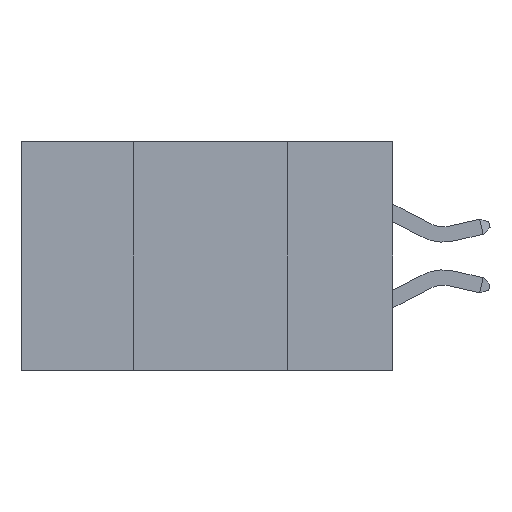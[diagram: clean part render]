
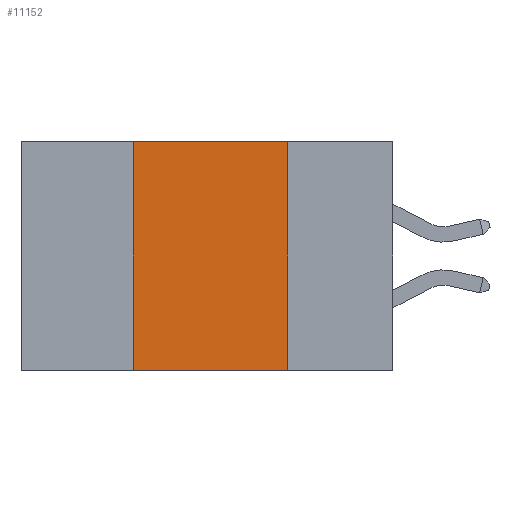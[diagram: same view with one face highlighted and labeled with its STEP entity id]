
A CAD part, left-side view. The second image highlights one B-rep face of the part: STEP entity #11152.
In plain terms, the highlighted planar face has unit normal (-1, 0, 0).
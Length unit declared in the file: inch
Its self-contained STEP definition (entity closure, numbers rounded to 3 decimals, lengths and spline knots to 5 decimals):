
#495 = DIRECTION ( 'NONE',  ( 0., 0., -1. ) ) ;
#962 = DIRECTION ( 'NONE',  ( 0., -1., 0. ) ) ;
#2037 = VECTOR ( 'NONE', #962, 39.37008 ) ;
#3722 = CARTESIAN_POINT ( 'NONE',  ( 0., 0.17, -0.37 ) ) ;
#4074 = ORIENTED_EDGE ( 'NONE', *, *, #23182, .F. ) ;
#4341 = VERTEX_POINT ( 'NONE', #3722 ) ;
#6495 = CARTESIAN_POINT ( 'NONE',  ( 0., 0.42, 0. ) ) ;
#6790 = LINE ( 'NONE', #6495, #18582 ) ;
#7471 = CARTESIAN_POINT ( 'NONE',  ( 0., 0.6, 0. ) ) ;
#7876 = VERTEX_POINT ( 'NONE', #23951 ) ;
#8425 = DIRECTION ( 'NONE',  ( 0., 0., -1. ) ) ;
#10256 = VERTEX_POINT ( 'NONE', #17752 ) ;
#10560 = LINE ( 'NONE', #11004, #13481 ) ;
#10595 = CARTESIAN_POINT ( 'NONE',  ( 0., 0.6, 0. ) ) ;
#11004 = CARTESIAN_POINT ( 'NONE',  ( 0., 0.6, -0.37 ) ) ;
#11152 = ADVANCED_FACE ( 'NONE', ( #28381 ), #21589, .F. ) ;
#11482 = CARTESIAN_POINT ( 'NONE',  ( 0., 0.17, 0. ) ) ;
#11497 = EDGE_CURVE ( 'NONE', #22914, #4341, #10560, .T. ) ;
#12917 = DIRECTION ( 'NONE',  ( 1., 0., 0. ) ) ;
#13481 = VECTOR ( 'NONE', #24138, 39.37008 ) ;
#13621 = EDGE_CURVE ( 'NONE', #7876, #10256, #27273, .T. ) ;
#16642 = ORIENTED_EDGE ( 'NONE', *, *, #11497, .T. ) ;
#17293 = VECTOR ( 'NONE', #495, 39.37008 ) ;
#17752 = CARTESIAN_POINT ( 'NONE',  ( 0., 0.17, 0. ) ) ;
#18126 = LINE ( 'NONE', #11482, #17293 ) ;
#18572 = CARTESIAN_POINT ( 'NONE',  ( 0., 0.42, -0.37 ) ) ;
#18582 = VECTOR ( 'NONE', #20209, 39.37008 ) ;
#20087 = ORIENTED_EDGE ( 'NONE', *, *, #25776, .F. ) ;
#20209 = DIRECTION ( 'NONE',  ( 0., 0., 1. ) ) ;
#21236 = EDGE_LOOP ( 'NONE', ( #4074, #22915, #20087, #16642 ) ) ;
#21589 = PLANE ( 'NONE',  #27912 ) ;
#22914 = VERTEX_POINT ( 'NONE', #18572 ) ;
#22915 = ORIENTED_EDGE ( 'NONE', *, *, #13621, .F. ) ;
#23182 = EDGE_CURVE ( 'NONE', #10256, #4341, #18126, .T. ) ;
#23951 = CARTESIAN_POINT ( 'NONE',  ( 0., 0.42, 0. ) ) ;
#24138 = DIRECTION ( 'NONE',  ( 0., -1., 0. ) ) ;
#25776 = EDGE_CURVE ( 'NONE', #22914, #7876, #6790, .T. ) ;
#27273 = LINE ( 'NONE', #7471, #2037 ) ;
#27912 = AXIS2_PLACEMENT_3D ( 'NONE', #10595, #12917, #8425 ) ;
#28381 = FACE_OUTER_BOUND ( 'NONE', #21236, .T. ) ;
